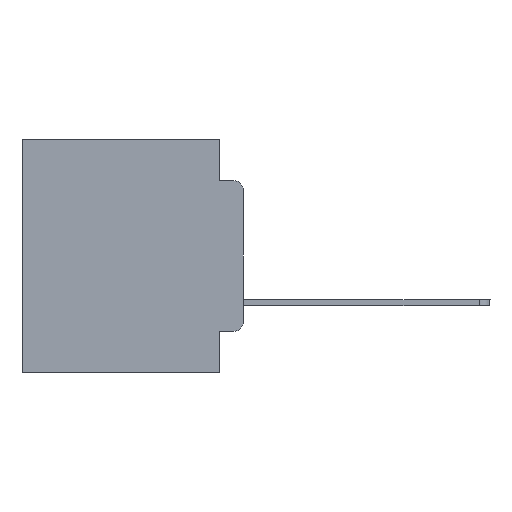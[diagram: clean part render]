
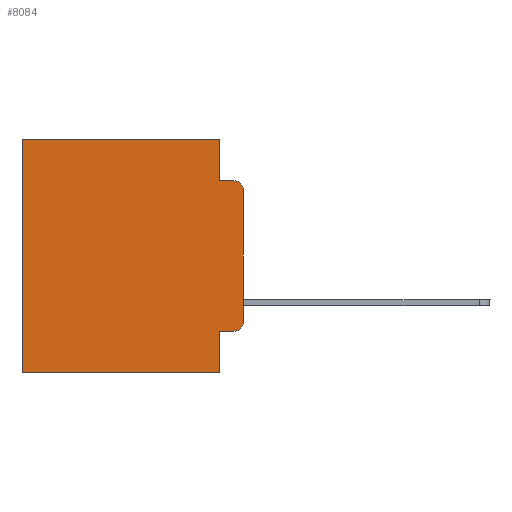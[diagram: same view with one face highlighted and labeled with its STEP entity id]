
A CAD part, left-side view. The second image highlights one B-rep face of the part: STEP entity #8084.
In plain terms, the highlighted planar face has unit normal (-1, 0, 0).
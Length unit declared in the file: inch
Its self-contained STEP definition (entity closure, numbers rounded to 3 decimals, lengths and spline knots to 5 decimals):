
#517 = VERTEX_POINT ( 'NONE', #18669 ) ;
#598 = DIRECTION ( 'NONE',  ( 0., 0., -1. ) ) ;
#849 = VERTEX_POINT ( 'NONE', #1520 ) ;
#1229 = VECTOR ( 'NONE', #11005, 39.37008 ) ;
#1520 = CARTESIAN_POINT ( 'NONE',  ( 0.298, 0.051, 0. ) ) ;
#1811 = ORIENTED_EDGE ( 'NONE', *, *, #3664, .T. ) ;
#1853 = CARTESIAN_POINT ( 'NONE',  ( 0.298, 0., -0.3915 ) ) ;
#1897 = AXIS2_PLACEMENT_3D ( 'NONE', #6849, #2371, #17621 ) ;
#2371 = DIRECTION ( 'NONE',  ( -1., 0., 0. ) ) ;
#2819 = CARTESIAN_POINT ( 'NONE',  ( 0.298, 0., 0. ) ) ;
#2892 = VERTEX_POINT ( 'NONE', #20638 ) ;
#3664 = EDGE_CURVE ( 'NONE', #2892, #517, #13026, .T. ) ;
#4209 = DIRECTION ( 'NONE',  ( 0., 1., 0. ) ) ;
#5250 = DIRECTION ( 'NONE',  ( 0., 0., -1. ) ) ;
#5664 = LINE ( 'NONE', #25965, #16569 ) ;
#6204 = LINE ( 'NONE', #20628, #10634 ) ;
#6534 = VECTOR ( 'NONE', #4209, 39.37008 ) ;
#6849 = CARTESIAN_POINT ( 'NONE',  ( 0.298, 0.02, -0.1085 ) ) ;
#7294 = VECTOR ( 'NONE', #20940, 39.37008 ) ;
#7603 = EDGE_CURVE ( 'NONE', #9879, #8547, #20298, .T. ) ;
#7650 = DIRECTION ( 'NONE',  ( 0., 0., -1. ) ) ;
#7772 = CARTESIAN_POINT ( 'NONE',  ( 0.298, 0.051, -0.0885 ) ) ;
#8084 = ADVANCED_FACE ( 'NONE', ( #15946 ), #11312, .F. ) ;
#8189 = DIRECTION ( 'NONE',  ( 0., 0., -1. ) ) ;
#8547 = VERTEX_POINT ( 'NONE', #1853 ) ;
#8903 = ORIENTED_EDGE ( 'NONE', *, *, #26380, .T. ) ;
#9549 = VERTEX_POINT ( 'NONE', #20649 ) ;
#9879 = VERTEX_POINT ( 'NONE', #26551 ) ;
#10615 = ORIENTED_EDGE ( 'NONE', *, *, #11944, .T. ) ;
#10634 = VECTOR ( 'NONE', #7650, 39.37008 ) ;
#11005 = DIRECTION ( 'NONE',  ( 0., 1., 0. ) ) ;
#11312 = PLANE ( 'NONE',  #12041 ) ;
#11767 = EDGE_CURVE ( 'NONE', #13374, #517, #20494, .T. ) ;
#11775 = ORIENTED_EDGE ( 'NONE', *, *, #14961, .F. ) ;
#11944 = EDGE_CURVE ( 'NONE', #14655, #27355, #17414, .T. ) ;
#12041 = AXIS2_PLACEMENT_3D ( 'NONE', #2819, #26880, #598 ) ;
#12062 = VECTOR ( 'NONE', #25546, 39.37008 ) ;
#12184 = ORIENTED_EDGE ( 'NONE', *, *, #11767, .F. ) ;
#12762 = CARTESIAN_POINT ( 'NONE',  ( 0.298, 0.051, -0.4115 ) ) ;
#13026 = LINE ( 'NONE', #23792, #14740 ) ;
#13374 = VERTEX_POINT ( 'NONE', #28286 ) ;
#13375 = ORIENTED_EDGE ( 'NONE', *, *, #7603, .T. ) ;
#14090 = VERTEX_POINT ( 'NONE', #12762 ) ;
#14494 = LINE ( 'NONE', #7772, #7294 ) ;
#14655 = VERTEX_POINT ( 'NONE', #16110 ) ;
#14682 = ORIENTED_EDGE ( 'NONE', *, *, #16201, .T. ) ;
#14696 = CARTESIAN_POINT ( 'NONE',  ( 0.298, 0.051, 0. ) ) ;
#14740 = VECTOR ( 'NONE', #15094, 39.37008 ) ;
#14961 = EDGE_CURVE ( 'NONE', #14655, #8547, #5664, .T. ) ;
#15094 = DIRECTION ( 'NONE',  ( 0., 0., -1. ) ) ;
#15483 = LINE ( 'NONE', #25731, #12062 ) ;
#15549 = EDGE_LOOP ( 'NONE', ( #11775, #10615, #25421, #19262, #8903, #1811, #12184, #23182, #14682, #13375 ) ) ;
#15946 = FACE_OUTER_BOUND ( 'NONE', #15549, .T. ) ;
#16110 = CARTESIAN_POINT ( 'NONE',  ( 0.298, 0., -0.1085 ) ) ;
#16201 = EDGE_CURVE ( 'NONE', #14090, #9879, #15483, .T. ) ;
#16370 = CARTESIAN_POINT ( 'NONE',  ( 0.298, 0.02, -0.0885 ) ) ;
#16419 = AXIS2_PLACEMENT_3D ( 'NONE', #26821, #24801, #5250 ) ;
#16569 = VECTOR ( 'NONE', #17059, 39.37008 ) ;
#16714 = EDGE_CURVE ( 'NONE', #9549, #27355, #14494, .T. ) ;
#17059 = DIRECTION ( 'NONE',  ( 0., 0., -1. ) ) ;
#17414 = CIRCLE ( 'NONE', #1897, 0.02 ) ;
#17621 = DIRECTION ( 'NONE',  ( 0., 0., -1. ) ) ;
#18669 = CARTESIAN_POINT ( 'NONE',  ( 0.298, 0.473, -0.5 ) ) ;
#19133 = CARTESIAN_POINT ( 'NONE',  ( 0.298, 0., -0.5 ) ) ;
#19262 = ORIENTED_EDGE ( 'NONE', *, *, #19566, .F. ) ;
#19566 = EDGE_CURVE ( 'NONE', #849, #9549, #20766, .T. ) ;
#20298 = CIRCLE ( 'NONE', #16419, 0.02 ) ;
#20494 = LINE ( 'NONE', #19133, #6534 ) ;
#20628 = CARTESIAN_POINT ( 'NONE',  ( 0.298, 0.051, 0. ) ) ;
#20638 = CARTESIAN_POINT ( 'NONE',  ( 0.298, 0.473, 0. ) ) ;
#20649 = CARTESIAN_POINT ( 'NONE',  ( 0.298, 0.051, -0.0885 ) ) ;
#20766 = LINE ( 'NONE', #14696, #24867 ) ;
#20940 = DIRECTION ( 'NONE',  ( 0., -1., 0. ) ) ;
#22761 = EDGE_CURVE ( 'NONE', #14090, #13374, #6204, .T. ) ;
#23182 = ORIENTED_EDGE ( 'NONE', *, *, #22761, .F. ) ;
#23792 = CARTESIAN_POINT ( 'NONE',  ( 0.298, 0.473, 0. ) ) ;
#24115 = CARTESIAN_POINT ( 'NONE',  ( 0.298, 0., 0. ) ) ;
#24801 = DIRECTION ( 'NONE',  ( -1., 0., 0. ) ) ;
#24867 = VECTOR ( 'NONE', #8189, 39.37008 ) ;
#25421 = ORIENTED_EDGE ( 'NONE', *, *, #16714, .F. ) ;
#25546 = DIRECTION ( 'NONE',  ( 0., -1., 0. ) ) ;
#25731 = CARTESIAN_POINT ( 'NONE',  ( 0.298, 0.051, -0.4115 ) ) ;
#25833 = LINE ( 'NONE', #24115, #1229 ) ;
#25965 = CARTESIAN_POINT ( 'NONE',  ( 0.298, 0., 0. ) ) ;
#26380 = EDGE_CURVE ( 'NONE', #849, #2892, #25833, .T. ) ;
#26551 = CARTESIAN_POINT ( 'NONE',  ( 0.298, 0.02, -0.4115 ) ) ;
#26821 = CARTESIAN_POINT ( 'NONE',  ( 0.298, 0.02, -0.3915 ) ) ;
#26880 = DIRECTION ( 'NONE',  ( 1., 0., 0. ) ) ;
#27355 = VERTEX_POINT ( 'NONE', #16370 ) ;
#28286 = CARTESIAN_POINT ( 'NONE',  ( 0.298, 0.051, -0.5 ) ) ;
